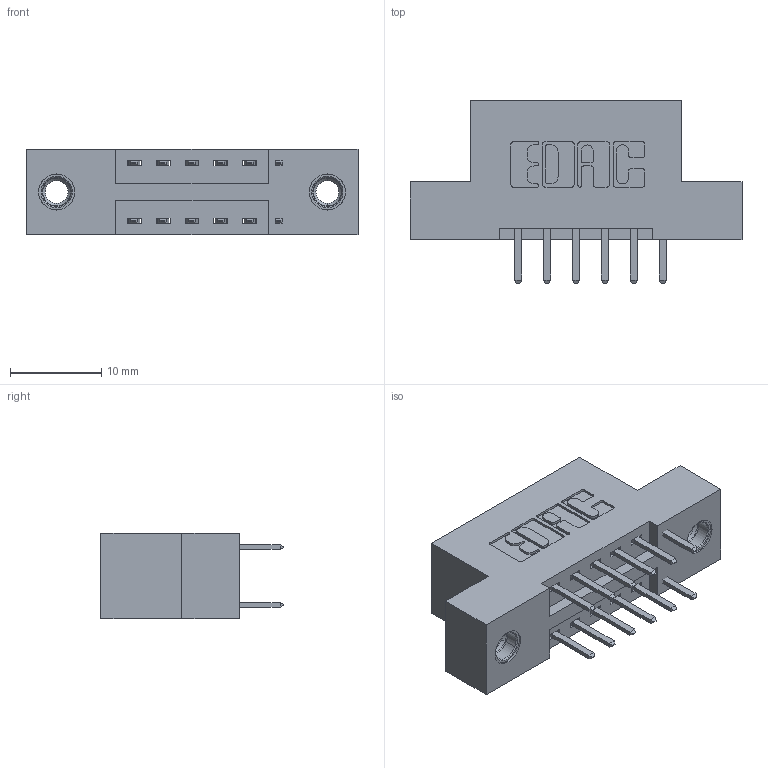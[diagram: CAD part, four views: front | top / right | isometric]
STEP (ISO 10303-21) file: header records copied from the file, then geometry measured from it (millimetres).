
FILE_DESCRIPTION (( 'STEP AP203' ), '1' );
FILE_NAME ('346-012-520-207.STEP', '2022-05-17T19:02:35', ( '' ), ( '' ), 'SwSTEP 2.0', 'SolidWorks 2020', '' );
FILE_SCHEMA (( 'CONFIG_CONTROL_DESIGN' ));
Length unit declared in the file: inch
Products named in the file (4): 345-250-001_345-250-005-103; 346 Part_Flush Mounting Lugs - 0.156 Dia-TI; 345-292-001_345-293-120; 346-012-520-207
Assembly tree (15 placements, depth 2):
  346-012-520-207
    346 Part_Flush Mounting Lugs - 0.156 Dia-TI
    345-292-001_345-293-120  x12
    345-250-001_345-250-005-103  x2
Bounding box: 36.45 x 20.02 x 9.4 mm (x, y, z)
Volume: 3266.1 mm3; surface area: 4033.1 mm2
Topology: 15 solids, 15 shells, 842 faces, 2379 edges, 1546 vertices
Faces by surface type: plane 542, cylinder 284, cone 12, torus 4
Entity records: 9608 total; most frequent: CARTESIAN_POINT 1621, ORIENTED_EDGE 1534, DIRECTION 1497, EDGE_CURVE 767, VECTOR 591, LINE 591, VERTEX_POINT 504, AXIS2_PLACEMENT_3D 453
